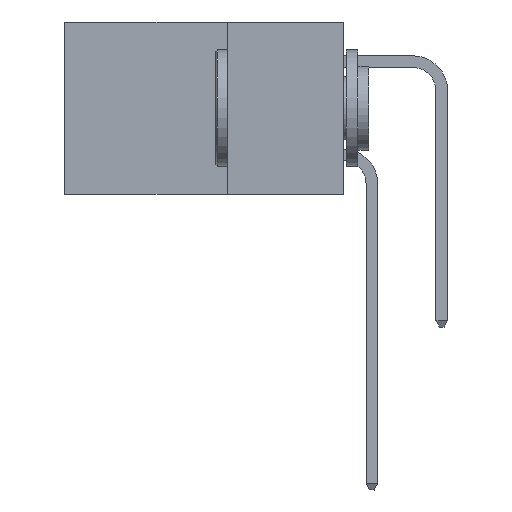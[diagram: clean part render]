
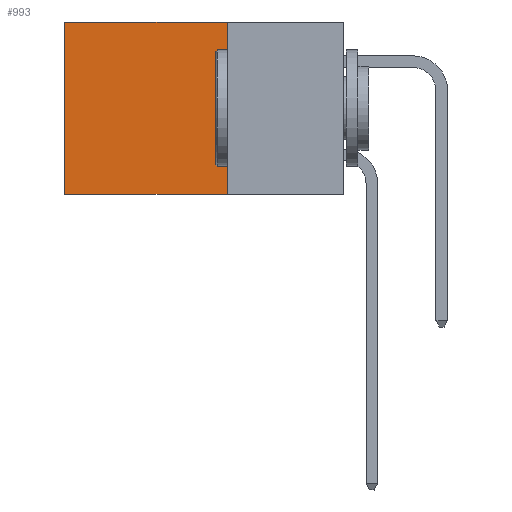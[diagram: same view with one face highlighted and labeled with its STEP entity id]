
A CAD part, left-side view. The second image highlights one B-rep face of the part: STEP entity #993.
In plain terms, the highlighted planar face has unit normal (-1, 0, 0).
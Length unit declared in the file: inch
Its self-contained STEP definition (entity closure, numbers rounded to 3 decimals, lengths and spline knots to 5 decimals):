
#147 = EDGE_CURVE ( 'NONE', #13303, #364, #6452, .T. ) ;
#364 = VERTEX_POINT ( 'NONE', #21105 ) ;
#366 = CARTESIAN_POINT ( 'NONE',  ( 0.298, 0.25, 0. ) ) ;
#993 = ADVANCED_FACE ( 'NONE', ( #9089 ), #2564, .F. ) ;
#2564 = PLANE ( 'NONE',  #25737 ) ;
#2786 = ORIENTED_EDGE ( 'NONE', *, *, #8225, .T. ) ;
#2835 = DIRECTION ( 'NONE',  ( 1., 0., 0. ) ) ;
#4465 = VECTOR ( 'NONE', #6782, 39.37008 ) ;
#6452 = LINE ( 'NONE', #13878, #15585 ) ;
#6782 = DIRECTION ( 'NONE',  ( 0., 0., -1. ) ) ;
#7259 = DIRECTION ( 'NONE',  ( 0., 1., 0. ) ) ;
#7756 = VECTOR ( 'NONE', #23255, 39.37008 ) ;
#8225 = EDGE_CURVE ( 'NONE', #364, #14021, #13495, .T. ) ;
#8726 = CARTESIAN_POINT ( 'NONE',  ( 0.298, 0.25, -0.37 ) ) ;
#9089 = FACE_OUTER_BOUND ( 'NONE', #9305, .T. ) ;
#9305 = EDGE_LOOP ( 'NONE', ( #2786, #22166, #14529, #23614 ) ) ;
#9334 = DIRECTION ( 'NONE',  ( 0., 0., -1. ) ) ;
#12870 = DIRECTION ( 'NONE',  ( 0., 1., 0. ) ) ;
#13303 = VERTEX_POINT ( 'NONE', #27880 ) ;
#13495 = LINE ( 'NONE', #25413, #7756 ) ;
#13591 = CARTESIAN_POINT ( 'NONE',  ( 0.298, 0.25, 0. ) ) ;
#13878 = CARTESIAN_POINT ( 'NONE',  ( 0.298, 0.25, 0. ) ) ;
#14021 = VERTEX_POINT ( 'NONE', #14954 ) ;
#14529 = ORIENTED_EDGE ( 'NONE', *, *, #21515, .F. ) ;
#14954 = CARTESIAN_POINT ( 'NONE',  ( 0.298, 0.6, -0.37 ) ) ;
#15585 = VECTOR ( 'NONE', #7259, 39.37008 ) ;
#21105 = CARTESIAN_POINT ( 'NONE',  ( 0.298, 0.6, 0. ) ) ;
#21515 = EDGE_CURVE ( 'NONE', #13303, #26877, #22680, .T. ) ;
#22166 = ORIENTED_EDGE ( 'NONE', *, *, #23301, .F. ) ;
#22680 = LINE ( 'NONE', #366, #4465 ) ;
#23255 = DIRECTION ( 'NONE',  ( 0., 0., -1. ) ) ;
#23301 = EDGE_CURVE ( 'NONE', #26877, #14021, #24609, .T. ) ;
#23614 = ORIENTED_EDGE ( 'NONE', *, *, #147, .T. ) ;
#24609 = LINE ( 'NONE', #27858, #26284 ) ;
#25413 = CARTESIAN_POINT ( 'NONE',  ( 0.298, 0.6, 0. ) ) ;
#25737 = AXIS2_PLACEMENT_3D ( 'NONE', #13591, #2835, #9334 ) ;
#26284 = VECTOR ( 'NONE', #12870, 39.37008 ) ;
#26877 = VERTEX_POINT ( 'NONE', #8726 ) ;
#27858 = CARTESIAN_POINT ( 'NONE',  ( 0.298, 0.25, -0.37 ) ) ;
#27880 = CARTESIAN_POINT ( 'NONE',  ( 0.298, 0.25, 0. ) ) ;
